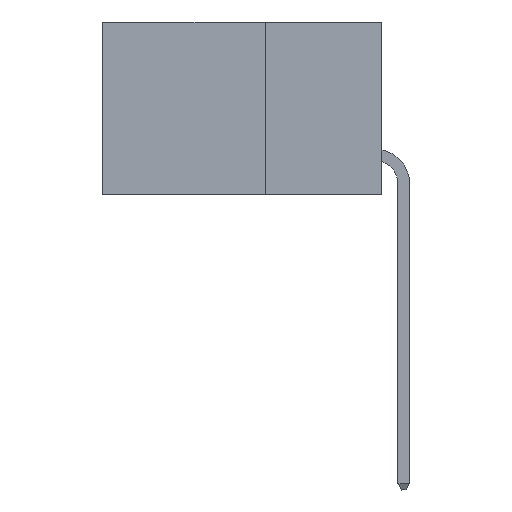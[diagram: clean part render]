
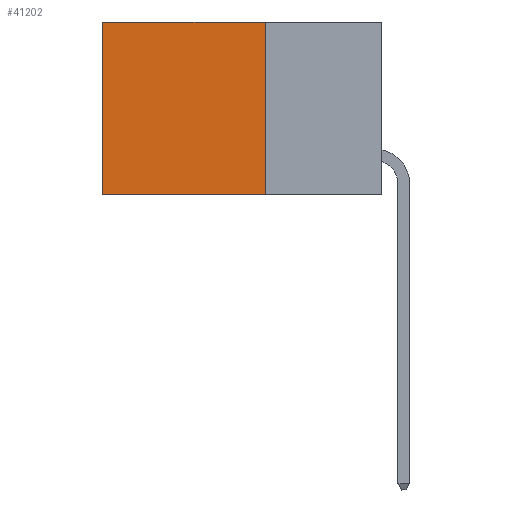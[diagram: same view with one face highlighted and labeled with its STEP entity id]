
A CAD part, left-side view. The second image highlights one B-rep face of the part: STEP entity #41202.
In plain terms, the highlighted planar face has unit normal (-1, 0, 0).
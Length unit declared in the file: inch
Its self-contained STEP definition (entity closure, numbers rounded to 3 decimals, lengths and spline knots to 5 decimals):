
#1258 = VECTOR ( 'NONE', #47690, 39.37008 ) ;
#2397 = CARTESIAN_POINT ( 'NONE',  ( 0.2875, 0.25, -0.37 ) ) ;
#3323 = DIRECTION ( 'NONE',  ( 0., 1., 0. ) ) ;
#6540 = DIRECTION ( 'NONE',  ( 0., 0., -1. ) ) ;
#7514 = LINE ( 'NONE', #17566, #16423 ) ;
#7730 = DIRECTION ( 'NONE',  ( 0., 1., 0. ) ) ;
#8585 = VERTEX_POINT ( 'NONE', #10881 ) ;
#8931 = ORIENTED_EDGE ( 'NONE', *, *, #41921, .T. ) ;
#9843 = LINE ( 'NONE', #20849, #17035 ) ;
#10881 = CARTESIAN_POINT ( 'NONE',  ( 0.2875, 0.6, 0. ) ) ;
#11473 = DIRECTION ( 'NONE',  ( 0., 0., -1. ) ) ;
#12768 = VERTEX_POINT ( 'NONE', #33552 ) ;
#14126 = AXIS2_PLACEMENT_3D ( 'NONE', #46292, #34432, #11473 ) ;
#14794 = FACE_OUTER_BOUND ( 'NONE', #29278, .T. ) ;
#16423 = VECTOR ( 'NONE', #6540, 39.37008 ) ;
#17035 = VECTOR ( 'NONE', #3323, 39.37008 ) ;
#17566 = CARTESIAN_POINT ( 'NONE',  ( 0.2875, 0.6, 0. ) ) ;
#17637 = VECTOR ( 'NONE', #7730, 39.37008 ) ;
#19563 = ORIENTED_EDGE ( 'NONE', *, *, #32882, .F. ) ;
#20849 = CARTESIAN_POINT ( 'NONE',  ( 0.2875, 0.25, 0. ) ) ;
#22649 = CARTESIAN_POINT ( 'NONE',  ( 0.2875, 0.25, -0.37 ) ) ;
#23622 = PLANE ( 'NONE',  #14126 ) ;
#25286 = EDGE_CURVE ( 'NONE', #46127, #8585, #9843, .T. ) ;
#25415 = LINE ( 'NONE', #22649, #17637 ) ;
#26484 = LINE ( 'NONE', #32271, #1258 ) ;
#27176 = CARTESIAN_POINT ( 'NONE',  ( 0.2875, 0.25, 0. ) ) ;
#29278 = EDGE_LOOP ( 'NONE', ( #8931, #39854, #19563, #42414 ) ) ;
#32271 = CARTESIAN_POINT ( 'NONE',  ( 0.2875, 0.25, 0. ) ) ;
#32882 = EDGE_CURVE ( 'NONE', #46127, #45773, #26484, .T. ) ;
#33552 = CARTESIAN_POINT ( 'NONE',  ( 0.2875, 0.6, -0.37 ) ) ;
#34432 = DIRECTION ( 'NONE',  ( 1., 0., 0. ) ) ;
#39854 = ORIENTED_EDGE ( 'NONE', *, *, #47530, .F. ) ;
#41202 = ADVANCED_FACE ( 'NONE', ( #14794 ), #23622, .F. ) ;
#41921 = EDGE_CURVE ( 'NONE', #8585, #12768, #7514, .T. ) ;
#42414 = ORIENTED_EDGE ( 'NONE', *, *, #25286, .T. ) ;
#45773 = VERTEX_POINT ( 'NONE', #2397 ) ;
#46127 = VERTEX_POINT ( 'NONE', #27176 ) ;
#46292 = CARTESIAN_POINT ( 'NONE',  ( 0.2875, 0.25, 0. ) ) ;
#47530 = EDGE_CURVE ( 'NONE', #45773, #12768, #25415, .T. ) ;
#47690 = DIRECTION ( 'NONE',  ( 0., 0., -1. ) ) ;
